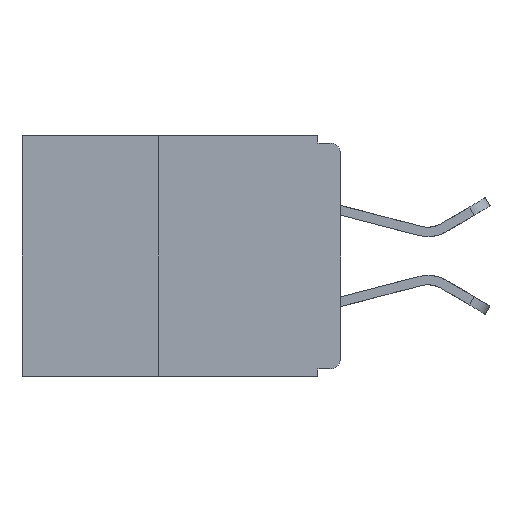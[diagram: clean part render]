
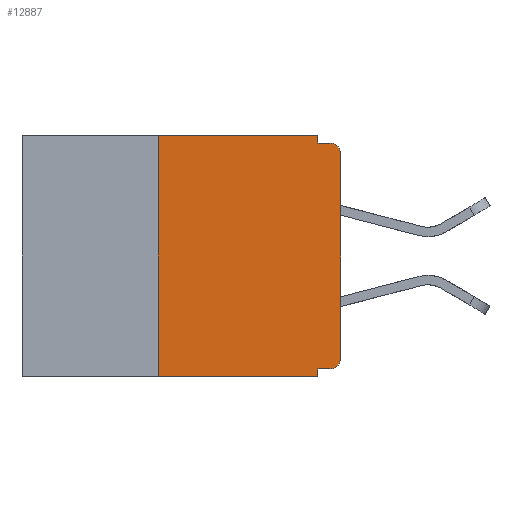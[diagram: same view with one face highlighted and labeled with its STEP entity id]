
A CAD part, left-side view. The second image highlights one B-rep face of the part: STEP entity #12887.
In plain terms, the highlighted planar face has unit normal (-1, 0, 0).
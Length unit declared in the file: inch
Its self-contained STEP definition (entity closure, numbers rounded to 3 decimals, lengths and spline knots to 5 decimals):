
#13 = AXIS2_PLACEMENT_3D ( 'NONE', #16870, #6588, #18589 ) ;
#233 = ORIENTED_EDGE ( 'NONE', *, *, #16075, .F. ) ;
#357 = VERTEX_POINT ( 'NONE', #8222 ) ;
#478 = DIRECTION ( 'NONE',  ( 0., 0., 1. ) ) ;
#484 = DIRECTION ( 'NONE',  ( 0., 0., -1. ) ) ;
#491 = ORIENTED_EDGE ( 'NONE', *, *, #11695, .T. ) ;
#530 = CARTESIAN_POINT ( 'NONE',  ( 0., 0., -0.305 ) ) ;
#805 = CARTESIAN_POINT ( 'NONE',  ( 0., 0., -0.32 ) ) ;
#883 = DIRECTION ( 'NONE',  ( 0., 1., 0. ) ) ;
#1197 = VECTOR ( 'NONE', #6815, 39.37008 ) ;
#1311 = DIRECTION ( 'NONE',  ( 0., -1., 0. ) ) ;
#1405 = AXIS2_PLACEMENT_3D ( 'NONE', #6508, #6483, #6477 ) ;
#1442 = VECTOR ( 'NONE', #3086, 39.37008 ) ;
#1461 = EDGE_CURVE ( 'NONE', #5395, #19322, #22179, .T. ) ;
#1756 = CARTESIAN_POINT ( 'NONE',  ( 0., 0.437, -0.33 ) ) ;
#2311 = DIRECTION ( 'NONE',  ( 0., 0., -1. ) ) ;
#2432 = VERTEX_POINT ( 'NONE', #7774 ) ;
#2491 = AXIS2_PLACEMENT_3D ( 'NONE', #3668, #15767, #5445 ) ;
#2693 = EDGE_CURVE ( 'NONE', #357, #5281, #20288, .T. ) ;
#2800 = VECTOR ( 'NONE', #13932, 39.37008 ) ;
#3059 = CARTESIAN_POINT ( 'NONE',  ( 0., 0.031, 0. ) ) ;
#3070 = CARTESIAN_POINT ( 'NONE',  ( 0., 0.437, 0. ) ) ;
#3086 = DIRECTION ( 'NONE',  ( 0., 0., 1. ) ) ;
#3668 = CARTESIAN_POINT ( 'NONE',  ( 0., 0.015, -0.305 ) ) ;
#3773 = LINE ( 'NONE', #21154, #22027 ) ;
#4110 = EDGE_CURVE ( 'NONE', #5397, #14795, #7425, .T. ) ;
#4472 = ORIENTED_EDGE ( 'NONE', *, *, #1461, .F. ) ;
#5230 = VECTOR ( 'NONE', #883, 39.37008 ) ;
#5255 = EDGE_LOOP ( 'NONE', ( #491, #7845, #8238, #4472, #233, #18174, #14040, #12538, #21715, #17833 ) ) ;
#5281 = VERTEX_POINT ( 'NONE', #13463 ) ;
#5395 = VERTEX_POINT ( 'NONE', #20603 ) ;
#5397 = VERTEX_POINT ( 'NONE', #8686 ) ;
#5445 = DIRECTION ( 'NONE',  ( 0., 0., -1. ) ) ;
#5882 = LINE ( 'NONE', #10234, #1197 ) ;
#6477 = DIRECTION ( 'NONE',  ( 0., 0., -1. ) ) ;
#6483 = DIRECTION ( 'NONE',  ( -1., 0., 0. ) ) ;
#6508 = CARTESIAN_POINT ( 'NONE',  ( 0., 0.015, -0.025 ) ) ;
#6588 = DIRECTION ( 'NONE',  ( 1., 0., 0. ) ) ;
#6815 = DIRECTION ( 'NONE',  ( 0., -1., 0. ) ) ;
#6957 = LINE ( 'NONE', #1756, #2800 ) ;
#7425 = CIRCLE ( 'NONE', #1405, 0.015 ) ;
#7774 = CARTESIAN_POINT ( 'NONE',  ( 0., 0.25, -0.33 ) ) ;
#7845 = ORIENTED_EDGE ( 'NONE', *, *, #4110, .T. ) ;
#7948 = EDGE_CURVE ( 'NONE', #16804, #357, #9853, .T. ) ;
#8222 = CARTESIAN_POINT ( 'NONE',  ( 0., 0.031, -0.32 ) ) ;
#8238 = ORIENTED_EDGE ( 'NONE', *, *, #16799, .F. ) ;
#8686 = CARTESIAN_POINT ( 'NONE',  ( 0., 0., -0.025 ) ) ;
#9114 = VERTEX_POINT ( 'NONE', #530 ) ;
#9241 = CIRCLE ( 'NONE', #2491, 0.015 ) ;
#9556 = EDGE_CURVE ( 'NONE', #16804, #9114, #9241, .T. ) ;
#9853 = LINE ( 'NONE', #805, #5230 ) ;
#10234 = CARTESIAN_POINT ( 'NONE',  ( 0., 0., -0.01 ) ) ;
#11044 = VERTEX_POINT ( 'NONE', #21831 ) ;
#11695 = EDGE_CURVE ( 'NONE', #9114, #5397, #15269, .T. ) ;
#11875 = EDGE_CURVE ( 'NONE', #2432, #5281, #6957, .T. ) ;
#12395 = VECTOR ( 'NONE', #1311, 39.37008 ) ;
#12538 = ORIENTED_EDGE ( 'NONE', *, *, #2693, .F. ) ;
#12887 = ADVANCED_FACE ( 'NONE', ( #13891 ), #21903, .F. ) ;
#13149 = VECTOR ( 'NONE', #2311, 39.37008 ) ;
#13463 = CARTESIAN_POINT ( 'NONE',  ( 0., 0.031, -0.33 ) ) ;
#13891 = FACE_OUTER_BOUND ( 'NONE', #5255, .T. ) ;
#13932 = DIRECTION ( 'NONE',  ( 0., -1., 0. ) ) ;
#14019 = EDGE_CURVE ( 'NONE', #2432, #11044, #3773, .T. ) ;
#14040 = ORIENTED_EDGE ( 'NONE', *, *, #11875, .T. ) ;
#14795 = VERTEX_POINT ( 'NONE', #19926 ) ;
#15269 = LINE ( 'NONE', #21941, #1442 ) ;
#15350 = CARTESIAN_POINT ( 'NONE',  ( 0., 0.031, -0.01 ) ) ;
#15767 = DIRECTION ( 'NONE',  ( -1., 0., 0. ) ) ;
#15769 = VECTOR ( 'NONE', #484, 39.37008 ) ;
#15962 = CARTESIAN_POINT ( 'NONE',  ( 0., 0.031, -0.33 ) ) ;
#16075 = EDGE_CURVE ( 'NONE', #11044, #5395, #16938, .T. ) ;
#16799 = EDGE_CURVE ( 'NONE', #19322, #14795, #5882, .T. ) ;
#16804 = VERTEX_POINT ( 'NONE', #18804 ) ;
#16870 = CARTESIAN_POINT ( 'NONE',  ( 0., 0.437, 0. ) ) ;
#16938 = LINE ( 'NONE', #3070, #12395 ) ;
#17833 = ORIENTED_EDGE ( 'NONE', *, *, #9556, .T. ) ;
#18174 = ORIENTED_EDGE ( 'NONE', *, *, #14019, .F. ) ;
#18589 = DIRECTION ( 'NONE',  ( 0., 0., -1. ) ) ;
#18804 = CARTESIAN_POINT ( 'NONE',  ( 0., 0.015, -0.32 ) ) ;
#19322 = VERTEX_POINT ( 'NONE', #15350 ) ;
#19926 = CARTESIAN_POINT ( 'NONE',  ( 0., 0.015, -0.01 ) ) ;
#20288 = LINE ( 'NONE', #15962, #15769 ) ;
#20603 = CARTESIAN_POINT ( 'NONE',  ( 0., 0.031, 0. ) ) ;
#21154 = CARTESIAN_POINT ( 'NONE',  ( 0., 0.25, -0.33 ) ) ;
#21715 = ORIENTED_EDGE ( 'NONE', *, *, #7948, .F. ) ;
#21831 = CARTESIAN_POINT ( 'NONE',  ( 0., 0.25, 0. ) ) ;
#21903 = PLANE ( 'NONE',  #13 ) ;
#21941 = CARTESIAN_POINT ( 'NONE',  ( 0., 0., 0. ) ) ;
#22027 = VECTOR ( 'NONE', #478, 39.37008 ) ;
#22179 = LINE ( 'NONE', #3059, #13149 ) ;
